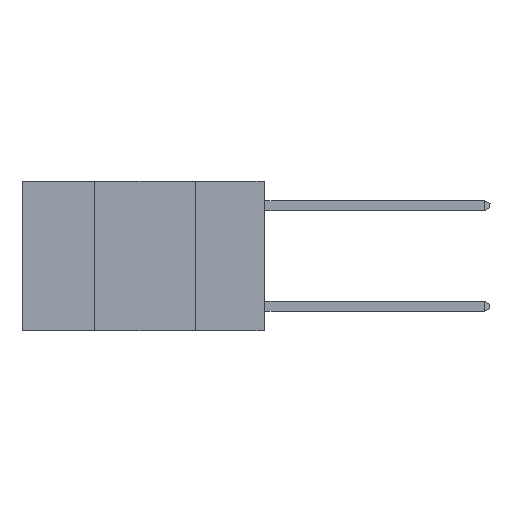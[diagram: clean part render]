
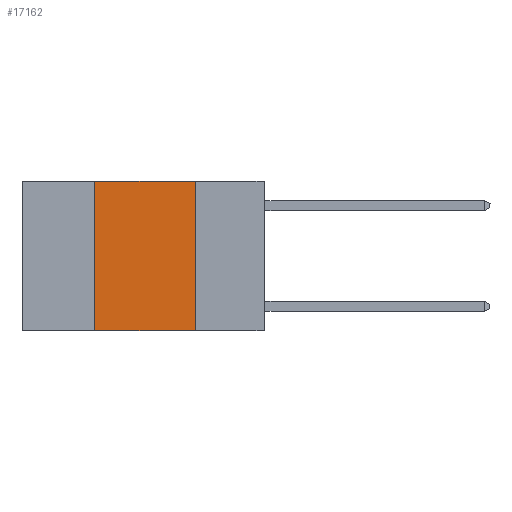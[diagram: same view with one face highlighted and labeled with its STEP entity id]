
A CAD part, left-side view. The second image highlights one B-rep face of the part: STEP entity #17162.
In plain terms, the highlighted planar face has unit normal (-1, 0, 0).
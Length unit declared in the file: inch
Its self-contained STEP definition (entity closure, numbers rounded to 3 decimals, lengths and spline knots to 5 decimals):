
#218 = PLANE ( 'NONE',  #17884 ) ;
#1031 = VERTEX_POINT ( 'NONE', #5523 ) ;
#1474 = LINE ( 'NONE', #14505, #9298 ) ;
#1588 = VERTEX_POINT ( 'NONE', #18306 ) ;
#3375 = DIRECTION ( 'NONE',  ( 0., 0., -1. ) ) ;
#4253 = VECTOR ( 'NONE', #18016, 39.37008 ) ;
#4481 = VECTOR ( 'NONE', #16006, 39.37008 ) ;
#5412 = EDGE_LOOP ( 'NONE', ( #13525, #6058, #15901, #6093 ) ) ;
#5523 = CARTESIAN_POINT ( 'NONE',  ( 0., 0.42, 0. ) ) ;
#5657 = VECTOR ( 'NONE', #10102, 39.37008 ) ;
#6058 = ORIENTED_EDGE ( 'NONE', *, *, #19334, .F. ) ;
#6093 = ORIENTED_EDGE ( 'NONE', *, *, #6474, .T. ) ;
#6472 = LINE ( 'NONE', #8360, #4253 ) ;
#6474 = EDGE_CURVE ( 'NONE', #1588, #18888, #1474, .T. ) ;
#7457 = EDGE_CURVE ( 'NONE', #1588, #1031, #15029, .T. ) ;
#8097 = CARTESIAN_POINT ( 'NONE',  ( 0., 0.6, 0. ) ) ;
#8360 = CARTESIAN_POINT ( 'NONE',  ( 0., 0.6, 0. ) ) ;
#9298 = VECTOR ( 'NONE', #19125, 39.37008 ) ;
#9952 = CARTESIAN_POINT ( 'NONE',  ( 0., 0.17, -0.37 ) ) ;
#10102 = DIRECTION ( 'NONE',  ( 0., 0., 1. ) ) ;
#11777 = FACE_OUTER_BOUND ( 'NONE', #5412, .T. ) ;
#13525 = ORIENTED_EDGE ( 'NONE', *, *, #15391, .F. ) ;
#14329 = CARTESIAN_POINT ( 'NONE',  ( 0., 0.17, 0. ) ) ;
#14505 = CARTESIAN_POINT ( 'NONE',  ( 0., 0.6, -0.37 ) ) ;
#15029 = LINE ( 'NONE', #16377, #5657 ) ;
#15391 = EDGE_CURVE ( 'NONE', #16486, #18888, #18970, .T. ) ;
#15901 = ORIENTED_EDGE ( 'NONE', *, *, #7457, .F. ) ;
#15904 = CARTESIAN_POINT ( 'NONE',  ( 0., 0.17, 0. ) ) ;
#16006 = DIRECTION ( 'NONE',  ( 0., 0., -1. ) ) ;
#16377 = CARTESIAN_POINT ( 'NONE',  ( 0., 0.42, 0. ) ) ;
#16486 = VERTEX_POINT ( 'NONE', #14329 ) ;
#17162 = ADVANCED_FACE ( 'NONE', ( #11777 ), #218, .F. ) ;
#17884 = AXIS2_PLACEMENT_3D ( 'NONE', #8097, #19451, #3375 ) ;
#18016 = DIRECTION ( 'NONE',  ( 0., -1., 0. ) ) ;
#18306 = CARTESIAN_POINT ( 'NONE',  ( 0., 0.42, -0.37 ) ) ;
#18888 = VERTEX_POINT ( 'NONE', #9952 ) ;
#18970 = LINE ( 'NONE', #15904, #4481 ) ;
#19125 = DIRECTION ( 'NONE',  ( 0., -1., 0. ) ) ;
#19334 = EDGE_CURVE ( 'NONE', #1031, #16486, #6472, .T. ) ;
#19451 = DIRECTION ( 'NONE',  ( 1., 0., 0. ) ) ;
